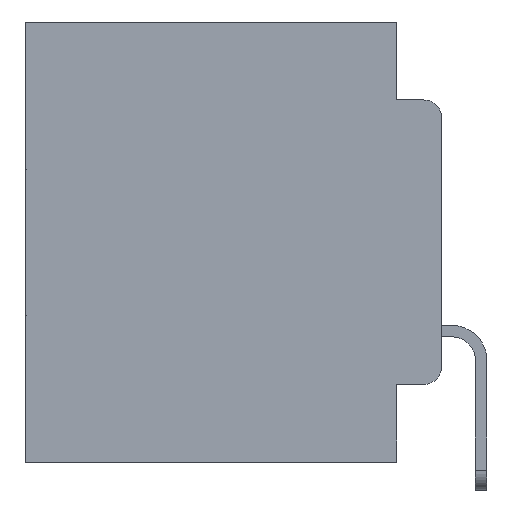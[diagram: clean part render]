
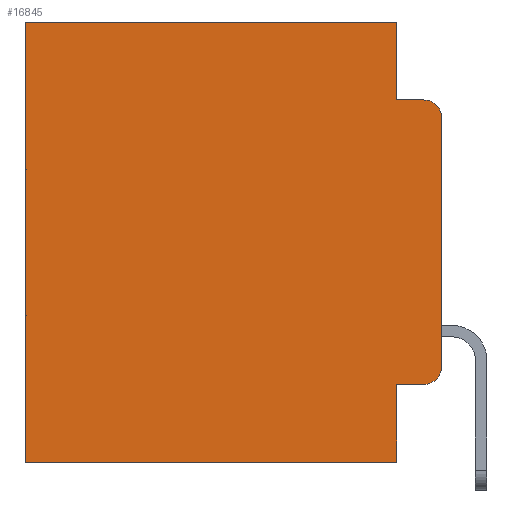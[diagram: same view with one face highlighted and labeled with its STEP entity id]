
A CAD part, left-side view. The second image highlights one B-rep face of the part: STEP entity #16845.
In plain terms, the highlighted planar face has unit normal (-1, 0, 0).
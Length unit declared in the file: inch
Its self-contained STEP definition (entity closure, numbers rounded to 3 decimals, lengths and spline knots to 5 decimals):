
#71 = ORIENTED_EDGE ( 'NONE', *, *, #10801, .T. ) ;
#297 = ORIENTED_EDGE ( 'NONE', *, *, #24362, .T. ) ;
#405 = VECTOR ( 'NONE', #3225, 39.37008 ) ;
#893 = LINE ( 'NONE', #17191, #25291 ) ;
#1813 = VERTEX_POINT ( 'NONE', #18200 ) ;
#2643 = CARTESIAN_POINT ( 'NONE',  ( 0.298, 0.051, 0. ) ) ;
#2901 = AXIS2_PLACEMENT_3D ( 'NONE', #24906, #11390, #26969 ) ;
#3225 = DIRECTION ( 'NONE',  ( 0., -1., 0. ) ) ;
#4336 = VERTEX_POINT ( 'NONE', #11015 ) ;
#4362 = EDGE_LOOP ( 'NONE', ( #13280, #5340, #10848, #7089, #5663, #6026, #9726, #9207, #297, #71 ) ) ;
#4556 = EDGE_CURVE ( 'NONE', #1813, #8998, #893, .T. ) ;
#4826 = LINE ( 'NONE', #24420, #27044 ) ;
#4846 = VERTEX_POINT ( 'NONE', #12315 ) ;
#5065 = DIRECTION ( 'NONE',  ( 0., -1., 0. ) ) ;
#5135 = CARTESIAN_POINT ( 'NONE',  ( 0.298, 0., 0. ) ) ;
#5164 = DIRECTION ( 'NONE',  ( 0., 0., -1. ) ) ;
#5197 = VECTOR ( 'NONE', #5065, 39.37008 ) ;
#5201 = EDGE_CURVE ( 'NONE', #4336, #13330, #19905, .T. ) ;
#5259 = AXIS2_PLACEMENT_3D ( 'NONE', #5135, #25900, #12478 ) ;
#5340 = ORIENTED_EDGE ( 'NONE', *, *, #25856, .T. ) ;
#5524 = CARTESIAN_POINT ( 'NONE',  ( 0.298, 0.02, -0.1085 ) ) ;
#5663 = ORIENTED_EDGE ( 'NONE', *, *, #29836, .T. ) ;
#5869 = CARTESIAN_POINT ( 'NONE',  ( 0.298, 0.02, -0.0885 ) ) ;
#5913 = DIRECTION ( 'NONE',  ( 0., 1., 0. ) ) ;
#6026 = ORIENTED_EDGE ( 'NONE', *, *, #9032, .T. ) ;
#6159 = VERTEX_POINT ( 'NONE', #6673 ) ;
#6336 = VECTOR ( 'NONE', #22572, 39.37008 ) ;
#6410 = CIRCLE ( 'NONE', #2901, 0.02 ) ;
#6673 = CARTESIAN_POINT ( 'NONE',  ( 0.298, 0., -0.1085 ) ) ;
#6756 = FACE_OUTER_BOUND ( 'NONE', #4362, .T. ) ;
#7089 = ORIENTED_EDGE ( 'NONE', *, *, #16433, .F. ) ;
#8013 = DIRECTION ( 'NONE',  ( 0., 0., -1. ) ) ;
#8639 = CARTESIAN_POINT ( 'NONE',  ( 0.298, 0., 0. ) ) ;
#8764 = VECTOR ( 'NONE', #27908, 39.37008 ) ;
#8998 = VERTEX_POINT ( 'NONE', #28168 ) ;
#9032 = EDGE_CURVE ( 'NONE', #26106, #4846, #22984, .T. ) ;
#9039 = CARTESIAN_POINT ( 'NONE',  ( 0.298, 0., -0.3915 ) ) ;
#9207 = ORIENTED_EDGE ( 'NONE', *, *, #4556, .F. ) ;
#9561 = VERTEX_POINT ( 'NONE', #13665 ) ;
#9726 = ORIENTED_EDGE ( 'NONE', *, *, #29628, .F. ) ;
#10236 = DIRECTION ( 'NONE',  ( 0., 0., -1. ) ) ;
#10769 = VECTOR ( 'NONE', #22087, 39.37008 ) ;
#10801 = EDGE_CURVE ( 'NONE', #27695, #12307, #6410, .T. ) ;
#10848 = ORIENTED_EDGE ( 'NONE', *, *, #5201, .F. ) ;
#11015 = CARTESIAN_POINT ( 'NONE',  ( 0.298, 0.051, -0.0885 ) ) ;
#11240 = CARTESIAN_POINT ( 'NONE',  ( 0.298, 0.02, -0.4115 ) ) ;
#11390 = DIRECTION ( 'NONE',  ( -1., 0., 0. ) ) ;
#11713 = LINE ( 'NONE', #19381, #5197 ) ;
#12307 = VERTEX_POINT ( 'NONE', #9039 ) ;
#12315 = CARTESIAN_POINT ( 'NONE',  ( 0.298, 0.473, -0.5 ) ) ;
#12478 = DIRECTION ( 'NONE',  ( 0., 0., -1. ) ) ;
#13280 = ORIENTED_EDGE ( 'NONE', *, *, #17033, .F. ) ;
#13330 = VERTEX_POINT ( 'NONE', #5869 ) ;
#13665 = CARTESIAN_POINT ( 'NONE',  ( 0.298, 0.051, 0. ) ) ;
#15443 = CIRCLE ( 'NONE', #29291, 0.02 ) ;
#16433 = EDGE_CURVE ( 'NONE', #9561, #4336, #25116, .T. ) ;
#16845 = ADVANCED_FACE ( 'NONE', ( #6756 ), #23831, .F. ) ;
#17033 = EDGE_CURVE ( 'NONE', #6159, #12307, #18263, .T. ) ;
#17145 = CARTESIAN_POINT ( 'NONE',  ( 0.298, 0., -0.5 ) ) ;
#17191 = CARTESIAN_POINT ( 'NONE',  ( 0.298, 0.051, 0. ) ) ;
#17762 = CARTESIAN_POINT ( 'NONE',  ( 0.298, 0.051, -0.0885 ) ) ;
#18200 = CARTESIAN_POINT ( 'NONE',  ( 0.298, 0.051, -0.4115 ) ) ;
#18247 = CARTESIAN_POINT ( 'NONE',  ( 0.298, 0.473, 0. ) ) ;
#18263 = LINE ( 'NONE', #8639, #6336 ) ;
#19381 = CARTESIAN_POINT ( 'NONE',  ( 0.298, 0.051, -0.4115 ) ) ;
#19905 = LINE ( 'NONE', #17762, #405 ) ;
#22061 = DIRECTION ( 'NONE',  ( -1., 0., 0. ) ) ;
#22087 = DIRECTION ( 'NONE',  ( 0., 0., -1. ) ) ;
#22572 = DIRECTION ( 'NONE',  ( 0., 0., -1. ) ) ;
#22984 = LINE ( 'NONE', #24142, #10769 ) ;
#23831 = PLANE ( 'NONE',  #5259 ) ;
#24142 = CARTESIAN_POINT ( 'NONE',  ( 0.298, 0.473, 0. ) ) ;
#24362 = EDGE_CURVE ( 'NONE', #1813, #27695, #11713, .T. ) ;
#24420 = CARTESIAN_POINT ( 'NONE',  ( 0.298, 0., 0. ) ) ;
#24906 = CARTESIAN_POINT ( 'NONE',  ( 0.298, 0.02, -0.3915 ) ) ;
#25116 = LINE ( 'NONE', #2643, #29895 ) ;
#25291 = VECTOR ( 'NONE', #10236, 39.37008 ) ;
#25856 = EDGE_CURVE ( 'NONE', #6159, #13330, #15443, .T. ) ;
#25900 = DIRECTION ( 'NONE',  ( 1., 0., 0. ) ) ;
#26106 = VERTEX_POINT ( 'NONE', #18247 ) ;
#26755 = LINE ( 'NONE', #17145, #8764 ) ;
#26969 = DIRECTION ( 'NONE',  ( 0., 0., -1. ) ) ;
#27044 = VECTOR ( 'NONE', #5913, 39.37008 ) ;
#27695 = VERTEX_POINT ( 'NONE', #11240 ) ;
#27908 = DIRECTION ( 'NONE',  ( 0., 1., 0. ) ) ;
#28168 = CARTESIAN_POINT ( 'NONE',  ( 0.298, 0.051, -0.5 ) ) ;
#29291 = AXIS2_PLACEMENT_3D ( 'NONE', #5524, #22061, #8013 ) ;
#29628 = EDGE_CURVE ( 'NONE', #8998, #4846, #26755, .T. ) ;
#29836 = EDGE_CURVE ( 'NONE', #9561, #26106, #4826, .T. ) ;
#29895 = VECTOR ( 'NONE', #5164, 39.37008 ) ;
